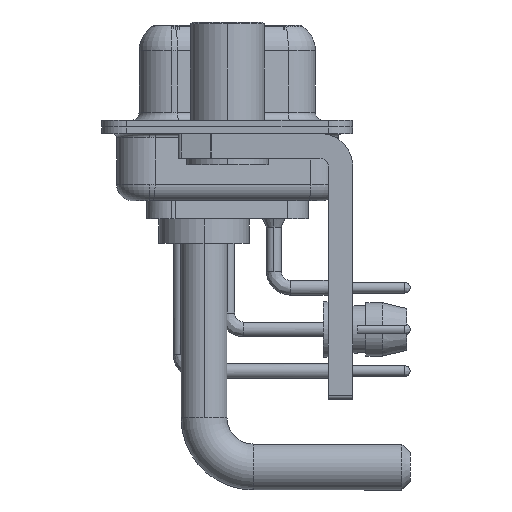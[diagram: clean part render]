
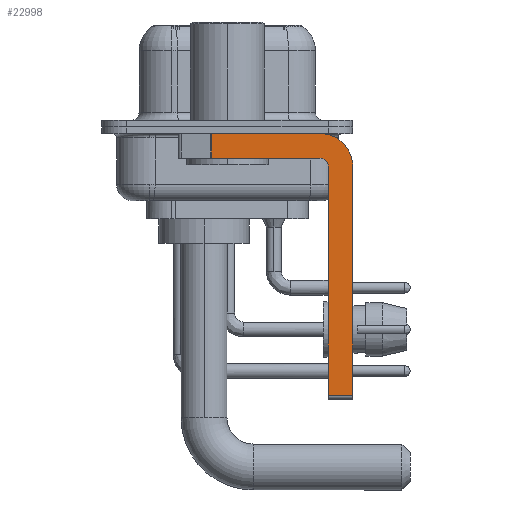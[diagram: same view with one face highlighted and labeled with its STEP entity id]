
A CAD part, left-side view. The second image highlights one B-rep face of the part: STEP entity #22998.
In plain terms, the highlighted planar face has unit normal (-1, 0, 0).
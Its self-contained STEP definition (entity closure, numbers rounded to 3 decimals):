
#281 = VERTEX_POINT ( 'NONE', #1128 ) ;
#1054 = VERTEX_POINT ( 'NONE', #15327 ) ;
#1128 = CARTESIAN_POINT ( 'NONE',  ( -2.9, -7.65, -2.4 ) ) ;
#1135 = EDGE_CURVE ( 'NONE', #25687, #281, #15528, .T. ) ;
#1191 = DIRECTION ( 'NONE',  ( 0., 0., -1. ) ) ;
#1331 = CARTESIAN_POINT ( 'NONE',  ( -2.9, -7.65, -2.4 ) ) ;
#2448 = VECTOR ( 'NONE', #29728, 1000. ) ;
#3007 = CARTESIAN_POINT ( 'NONE',  ( -2.9, -5.65, -1.9 ) ) ;
#3636 = VECTOR ( 'NONE', #10839, 1000. ) ;
#4385 = CARTESIAN_POINT ( 'NONE',  ( -2.9, -5.65, -2.4 ) ) ;
#4551 = PLANE ( 'NONE',  #18891 ) ;
#4933 = ORIENTED_EDGE ( 'NONE', *, *, #13496, .F. ) ;
#5185 = CARTESIAN_POINT ( 'NONE',  ( -2.9, -7.65, -16.35 ) ) ;
#7054 = DIRECTION ( 'NONE',  ( 0., 0., -1. ) ) ;
#7398 = CARTESIAN_POINT ( 'NONE',  ( -2.9, -6.15, -16.35 ) ) ;
#8161 = EDGE_CURVE ( 'NONE', #20030, #25687, #20411, .T. ) ;
#8321 = LINE ( 'NONE', #1331, #25842 ) ;
#8655 = DIRECTION ( 'NONE',  ( 0., 0., -1. ) ) ;
#9243 = DIRECTION ( 'NONE',  ( 0., 0., 1. ) ) ;
#9454 = ORIENTED_EDGE ( 'NONE', *, *, #13042, .T. ) ;
#9843 = ORIENTED_EDGE ( 'NONE', *, *, #20605, .F. ) ;
#10255 = VERTEX_POINT ( 'NONE', #5185 ) ;
#10839 = DIRECTION ( 'NONE',  ( 0., 1., 0. ) ) ;
#13042 = EDGE_CURVE ( 'NONE', #20030, #1054, #23536, .T. ) ;
#13055 = VERTEX_POINT ( 'NONE', #26009 ) ;
#13192 = AXIS2_PLACEMENT_3D ( 'NONE', #28287, #25460, #20640 ) ;
#13496 = EDGE_CURVE ( 'NONE', #281, #10255, #8321, .T. ) ;
#14085 = VECTOR ( 'NONE', #1191, 1000. ) ;
#14768 = DIRECTION ( 'NONE',  ( 0., -1., 0. ) ) ;
#15327 = CARTESIAN_POINT ( 'NONE',  ( -2.9, 0.978, -1.9 ) ) ;
#15528 = CIRCLE ( 'NONE', #28270, 2. ) ;
#15569 = ORIENTED_EDGE ( 'NONE', *, *, #8161, .F. ) ;
#16300 = DIRECTION ( 'NONE',  ( 0., 0., -1. ) ) ;
#17268 = VERTEX_POINT ( 'NONE', #7398 ) ;
#17905 = CARTESIAN_POINT ( 'NONE',  ( -2.9, 3., -0.4 ) ) ;
#18580 = ORIENTED_EDGE ( 'NONE', *, *, #25406, .T. ) ;
#18681 = CARTESIAN_POINT ( 'NONE',  ( -2.9, -5.65, -0.4 ) ) ;
#18891 = AXIS2_PLACEMENT_3D ( 'NONE', #4385, #29835, #7054 ) ;
#19542 = FACE_OUTER_BOUND ( 'NONE', #26104, .T. ) ;
#20030 = VERTEX_POINT ( 'NONE', #21016 ) ;
#20411 = LINE ( 'NONE', #17905, #23436 ) ;
#20605 = EDGE_CURVE ( 'NONE', #17268, #13055, #31516, .T. ) ;
#20640 = DIRECTION ( 'NONE',  ( 0., 0., 1. ) ) ;
#21016 = CARTESIAN_POINT ( 'NONE',  ( -2.9, 0.978, -0.4 ) ) ;
#22998 = ADVANCED_FACE ( 'NONE', ( #19542 ), #4551, .F. ) ;
#23436 = VECTOR ( 'NONE', #14768, 1000. ) ;
#23536 = LINE ( 'NONE', #30668, #14085 ) ;
#23555 = ORIENTED_EDGE ( 'NONE', *, *, #28833, .F. ) ;
#24349 = CARTESIAN_POINT ( 'NONE',  ( -2.9, -6.15, -16.6 ) ) ;
#24948 = ORIENTED_EDGE ( 'NONE', *, *, #28733, .F. ) ;
#25406 = EDGE_CURVE ( 'NONE', #17268, #10255, #32059, .T. ) ;
#25407 = CIRCLE ( 'NONE', #13192, 0.5 ) ;
#25460 = DIRECTION ( 'NONE',  ( -1., 0., 0. ) ) ;
#25687 = VERTEX_POINT ( 'NONE', #18681 ) ;
#25788 = LINE ( 'NONE', #3007, #3636 ) ;
#25842 = VECTOR ( 'NONE', #8655, 1000. ) ;
#26009 = CARTESIAN_POINT ( 'NONE',  ( -2.9, -6.15, -2.4 ) ) ;
#26104 = EDGE_LOOP ( 'NONE', ( #15569, #9454, #23555, #24948, #9843, #18580, #4933, #32383 ) ) ;
#26281 = CARTESIAN_POINT ( 'NONE',  ( -2.9, -5.65, -2.4 ) ) ;
#26596 = DIRECTION ( 'NONE',  ( 1., 0., 0. ) ) ;
#26712 = VERTEX_POINT ( 'NONE', #30912 ) ;
#28270 = AXIS2_PLACEMENT_3D ( 'NONE', #26281, #26596, #16300 ) ;
#28287 = CARTESIAN_POINT ( 'NONE',  ( -2.9, -5.65, -2.4 ) ) ;
#28733 = EDGE_CURVE ( 'NONE', #13055, #26712, #25407, .T. ) ;
#28833 = EDGE_CURVE ( 'NONE', #26712, #1054, #25788, .T. ) ;
#28952 = VECTOR ( 'NONE', #9243, 1000. ) ;
#29728 = DIRECTION ( 'NONE',  ( 0., -1., 0. ) ) ;
#29835 = DIRECTION ( 'NONE',  ( 1., 0., 0. ) ) ;
#30668 = CARTESIAN_POINT ( 'NONE',  ( -2.9, 0.978, -1.9 ) ) ;
#30912 = CARTESIAN_POINT ( 'NONE',  ( -2.9, -5.65, -1.9 ) ) ;
#31516 = LINE ( 'NONE', #24349, #28952 ) ;
#31728 = CARTESIAN_POINT ( 'NONE',  ( -2.9, -5.65, -16.35 ) ) ;
#32059 = LINE ( 'NONE', #31728, #2448 ) ;
#32383 = ORIENTED_EDGE ( 'NONE', *, *, #1135, .F. ) ;
